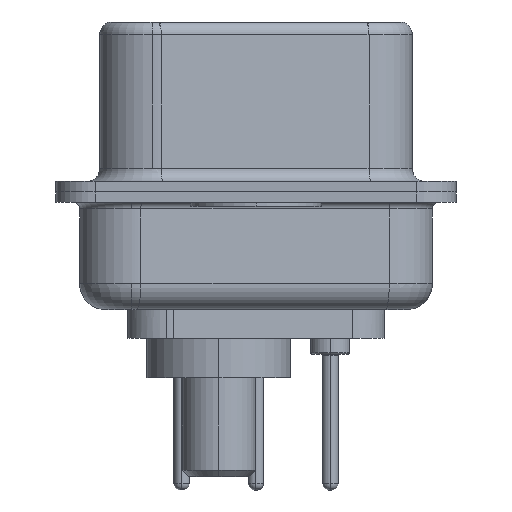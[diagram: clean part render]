
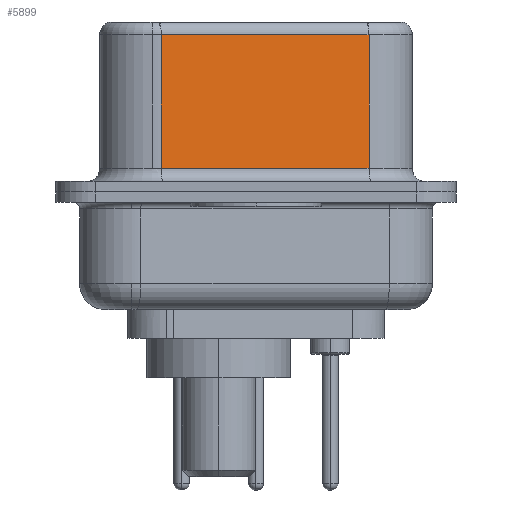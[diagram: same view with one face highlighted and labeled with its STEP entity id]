
A CAD part, left-side view. The second image highlights one B-rep face of the part: STEP entity #5899.
In plain terms, the highlighted planar face has unit normal (-0.985, -0.174, 0).
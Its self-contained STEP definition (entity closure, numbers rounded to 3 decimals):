
#281 = ORIENTED_EDGE ( 'NONE', *, *, #16636, .T. ) ;
#1090 = PLANE ( 'NONE',  #23522 ) ;
#1329 = VERTEX_POINT ( 'NONE', #24015 ) ;
#2351 = DIRECTION ( 'NONE',  ( 0.985, 0.174, 0. ) ) ;
#2974 = DIRECTION ( 'NONE',  ( -0.174, 0.985, 0. ) ) ;
#3374 = DIRECTION ( 'NONE',  ( 0., 0., -1. ) ) ;
#4775 = VECTOR ( 'NONE', #7654, 1000. ) ;
#5221 = VECTOR ( 'NONE', #12326, 1000. ) ;
#5352 = LINE ( 'NONE', #5745, #4775 ) ;
#5745 = CARTESIAN_POINT ( 'NONE',  ( 5.132, -4.322, 0.9 ) ) ;
#5756 = FACE_OUTER_BOUND ( 'NONE', #7185, .T. ) ;
#5899 = ADVANCED_FACE ( 'NONE', ( #5756 ), #1090, .F. ) ;
#6004 = ORIENTED_EDGE ( 'NONE', *, *, #14671, .F. ) ;
#6514 = VECTOR ( 'NONE', #15504, 1000. ) ;
#7185 = EDGE_LOOP ( 'NONE', ( #6004, #10792, #281, #18194 ) ) ;
#7654 = DIRECTION ( 'NONE',  ( 0.174, -0.985, 0. ) ) ;
#8927 = EDGE_CURVE ( 'NONE', #1329, #10485, #5352, .T. ) ;
#9706 = LINE ( 'NONE', #14222, #5221 ) ;
#10485 = VERTEX_POINT ( 'NONE', #14188 ) ;
#10792 = ORIENTED_EDGE ( 'NONE', *, *, #21894, .T. ) ;
#11604 = LINE ( 'NONE', #21062, #6514 ) ;
#12038 = LINE ( 'NONE', #12931, #21993 ) ;
#12326 = DIRECTION ( 'NONE',  ( 0., 0., -1. ) ) ;
#12843 = VERTEX_POINT ( 'NONE', #23584 ) ;
#12853 = CARTESIAN_POINT ( 'NONE',  ( 5.132, -4.322, 6.52 ) ) ;
#12931 = CARTESIAN_POINT ( 'NONE',  ( 5.132, -4.322, 6.52 ) ) ;
#14188 = CARTESIAN_POINT ( 'NONE',  ( 5.132, -4.322, 0.9 ) ) ;
#14222 = CARTESIAN_POINT ( 'NONE',  ( 3.73, 3.628, 6.52 ) ) ;
#14671 = EDGE_CURVE ( 'NONE', #12843, #10485, #12038, .T. ) ;
#15504 = DIRECTION ( 'NONE',  ( -0.174, 0.985, 0. ) ) ;
#16636 = EDGE_CURVE ( 'NONE', #22359, #1329, #9706, .T. ) ;
#18194 = ORIENTED_EDGE ( 'NONE', *, *, #8927, .T. ) ;
#18753 = CARTESIAN_POINT ( 'NONE',  ( 3.73, 3.628, 6.02 ) ) ;
#21062 = CARTESIAN_POINT ( 'NONE',  ( 5.132, -4.322, 6.02 ) ) ;
#21894 = EDGE_CURVE ( 'NONE', #12843, #22359, #11604, .T. ) ;
#21993 = VECTOR ( 'NONE', #3374, 1000. ) ;
#22359 = VERTEX_POINT ( 'NONE', #18753 ) ;
#23522 = AXIS2_PLACEMENT_3D ( 'NONE', #12853, #2351, #2974 ) ;
#23584 = CARTESIAN_POINT ( 'NONE',  ( 5.132, -4.322, 6.02 ) ) ;
#24015 = CARTESIAN_POINT ( 'NONE',  ( 3.73, 3.628, 0.9 ) ) ;
